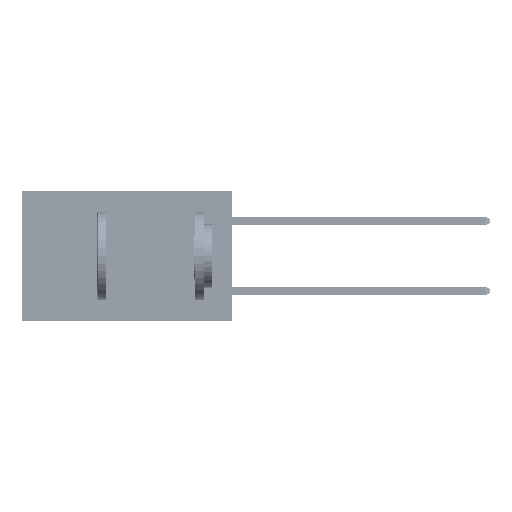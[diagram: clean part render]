
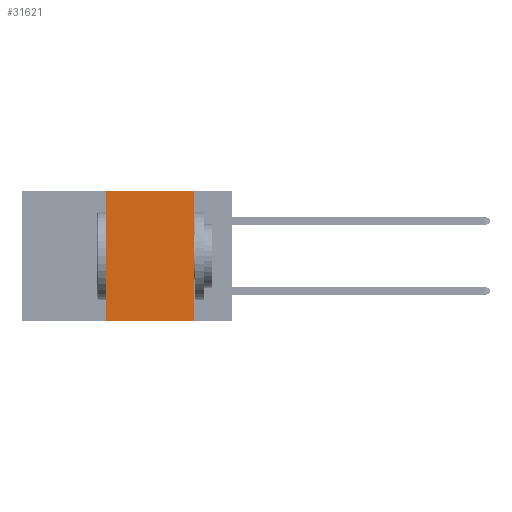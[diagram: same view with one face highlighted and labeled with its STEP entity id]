
A CAD part, left-side view. The second image highlights one B-rep face of the part: STEP entity #31621.
In plain terms, the highlighted planar face has unit normal (-1, 0, 0).
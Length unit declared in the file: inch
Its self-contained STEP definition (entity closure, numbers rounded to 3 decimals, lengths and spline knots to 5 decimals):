
#2271 = ORIENTED_EDGE ( 'NONE', *, *, #4499, .F. ) ;
#2541 = CARTESIAN_POINT ( 'NONE',  ( 0., 0.6, 0. ) ) ;
#4169 = DIRECTION ( 'NONE',  ( 0., -1., 0. ) ) ;
#4499 = EDGE_CURVE ( 'NONE', #21854, #46377, #6318, .T. ) ;
#4917 = ORIENTED_EDGE ( 'NONE', *, *, #13627, .F. ) ;
#6318 = LINE ( 'NONE', #24655, #34805 ) ;
#6869 = FACE_OUTER_BOUND ( 'NONE', #20801, .T. ) ;
#9941 = VECTOR ( 'NONE', #25086, 39.37008 ) ;
#10336 = ORIENTED_EDGE ( 'NONE', *, *, #18258, .T. ) ;
#12540 = DIRECTION ( 'NONE',  ( 0., 0., 1. ) ) ;
#13627 = EDGE_CURVE ( 'NONE', #21838, #21854, #22083, .T. ) ;
#15416 = AXIS2_PLACEMENT_3D ( 'NONE', #2541, #30900, #26465 ) ;
#16099 = LINE ( 'NONE', #31637, #50260 ) ;
#18258 = EDGE_CURVE ( 'NONE', #21838, #33315, #28900, .T. ) ;
#20292 = EDGE_CURVE ( 'NONE', #46377, #33315, #16099, .T. ) ;
#20801 = EDGE_LOOP ( 'NONE', ( #45403, #2271, #4917, #10336 ) ) ;
#20912 = CARTESIAN_POINT ( 'NONE',  ( 0., 0.36, -0.37 ) ) ;
#21838 = VERTEX_POINT ( 'NONE', #20912 ) ;
#21854 = VERTEX_POINT ( 'NONE', #24998 ) ;
#22083 = LINE ( 'NONE', #44766, #50566 ) ;
#23606 = DIRECTION ( 'NONE',  ( 0., 0., -1. ) ) ;
#24655 = CARTESIAN_POINT ( 'NONE',  ( 0., 0.6, 0. ) ) ;
#24998 = CARTESIAN_POINT ( 'NONE',  ( 0., 0.36, 0. ) ) ;
#25086 = DIRECTION ( 'NONE',  ( 0., -1., 0. ) ) ;
#26465 = DIRECTION ( 'NONE',  ( 0., 0., -1. ) ) ;
#27244 = CARTESIAN_POINT ( 'NONE',  ( 0., 0.11, 0. ) ) ;
#28900 = LINE ( 'NONE', #45801, #9941 ) ;
#29874 = CARTESIAN_POINT ( 'NONE',  ( 0., 0.11, -0.37 ) ) ;
#30396 = PLANE ( 'NONE',  #15416 ) ;
#30900 = DIRECTION ( 'NONE',  ( 1., 0., 0. ) ) ;
#31621 = ADVANCED_FACE ( 'NONE', ( #6869 ), #30396, .F. ) ;
#31637 = CARTESIAN_POINT ( 'NONE',  ( 0., 0.11, 0. ) ) ;
#33315 = VERTEX_POINT ( 'NONE', #29874 ) ;
#34805 = VECTOR ( 'NONE', #4169, 39.37008 ) ;
#44766 = CARTESIAN_POINT ( 'NONE',  ( 0., 0.36, 0. ) ) ;
#45403 = ORIENTED_EDGE ( 'NONE', *, *, #20292, .F. ) ;
#45801 = CARTESIAN_POINT ( 'NONE',  ( 0., 0.6, -0.37 ) ) ;
#46377 = VERTEX_POINT ( 'NONE', #27244 ) ;
#50260 = VECTOR ( 'NONE', #23606, 39.37008 ) ;
#50566 = VECTOR ( 'NONE', #12540, 39.37008 ) ;
